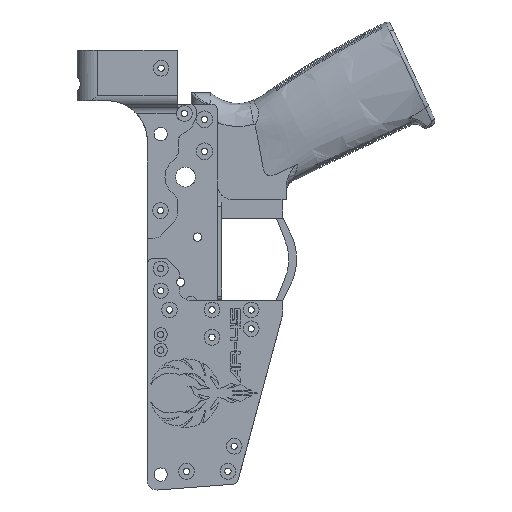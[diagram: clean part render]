
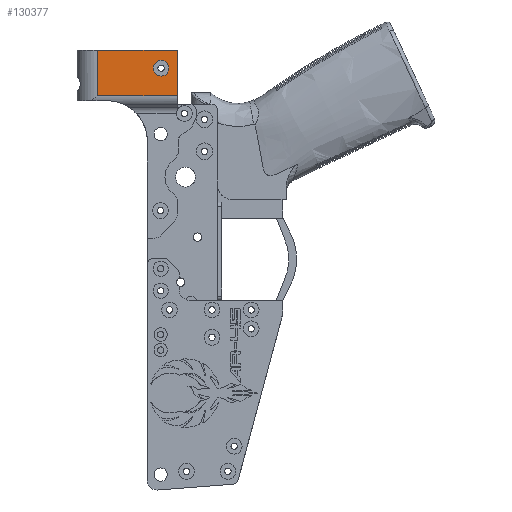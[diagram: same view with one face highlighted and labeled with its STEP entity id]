
A CAD part, left-side view. The second image highlights one B-rep face of the part: STEP entity #130377.
In plain terms, the highlighted planar face has unit normal (-1, 0, 0).
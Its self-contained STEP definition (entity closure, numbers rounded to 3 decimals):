
#2563 = CARTESIAN_POINT ( 'NONE',  ( -25., 7.678, -12.776 ) ) ;
#2951 = LINE ( 'NONE', #140693, #109962 ) ;
#7996 = EDGE_CURVE ( 'NONE', #59619, #16362, #136589, .T. ) ;
#9324 = AXIS2_PLACEMENT_3D ( 'NONE', #116725, #48260, #82517 ) ;
#12332 = EDGE_LOOP ( 'NONE', ( #117339, #46170 ) ) ;
#13072 = ORIENTED_EDGE ( 'NONE', *, *, #69360, .T. ) ;
#13967 = FACE_OUTER_BOUND ( 'NONE', #111401, .T. ) ;
#14723 = EDGE_CURVE ( 'NONE', #73125, #59619, #2951, .T. ) ;
#15175 = AXIS2_PLACEMENT_3D ( 'NONE', #59924, #96375, #49490 ) ;
#16362 = VERTEX_POINT ( 'NONE', #33906 ) ;
#18958 = CARTESIAN_POINT ( 'NONE',  ( -25., -30.202, -14.306 ) ) ;
#33906 = CARTESIAN_POINT ( 'NONE',  ( -25., 7.678, -10.291 ) ) ;
#35021 = CARTESIAN_POINT ( 'NONE',  ( -25., -22.502, 6.484 ) ) ;
#36368 = EDGE_CURVE ( 'NONE', #93127, #79195, #93649, .T. ) ;
#45684 = DIRECTION ( 'NONE',  ( -1., 0., 0. ) ) ;
#46170 = ORIENTED_EDGE ( 'NONE', *, *, #36368, .F. ) ;
#48260 = DIRECTION ( 'NONE',  ( 1., 0., 0. ) ) ;
#49490 = DIRECTION ( 'NONE',  ( 0., 0., 1. ) ) ;
#50831 = ORIENTED_EDGE ( 'NONE', *, *, #126546, .T. ) ;
#52582 = VECTOR ( 'NONE', #142627, 1000. ) ;
#58824 = VECTOR ( 'NONE', #123405, 1000. ) ;
#59619 = VERTEX_POINT ( 'NONE', #101866 ) ;
#59924 = CARTESIAN_POINT ( 'NONE',  ( -25., -22.502, 2.734 ) ) ;
#64695 = ORIENTED_EDGE ( 'NONE', *, *, #14723, .T. ) ;
#69360 = EDGE_CURVE ( 'NONE', #131514, #73125, #86780, .T. ) ;
#73125 = VERTEX_POINT ( 'NONE', #139478 ) ;
#76999 = DIRECTION ( 'NONE',  ( 0., 0., 1. ) ) ;
#79195 = VERTEX_POINT ( 'NONE', #35021 ) ;
#80540 = EDGE_CURVE ( 'NONE', #79195, #93127, #87482, .T. ) ;
#81036 = PLANE ( 'NONE',  #9324 ) ;
#82517 = DIRECTION ( 'NONE',  ( 0., 0., -1. ) ) ;
#86780 = LINE ( 'NONE', #18958, #52582 ) ;
#87482 = CIRCLE ( 'NONE', #111239, 3.75 ) ;
#90685 = CARTESIAN_POINT ( 'NONE',  ( -25., -36.779, -10.291 ) ) ;
#92203 = FACE_BOUND ( 'NONE', #12332, .T. ) ;
#93127 = VERTEX_POINT ( 'NONE', #114815 ) ;
#93431 = DIRECTION ( 'NONE',  ( 0., 0., -1. ) ) ;
#93649 = CIRCLE ( 'NONE', #15175, 3.75 ) ;
#96375 = DIRECTION ( 'NONE',  ( -1., 0., 0. ) ) ;
#101550 = ORIENTED_EDGE ( 'NONE', *, *, #7996, .T. ) ;
#101866 = CARTESIAN_POINT ( 'NONE',  ( -25., 7.678, 11.224 ) ) ;
#102276 = CARTESIAN_POINT ( 'NONE',  ( -25., -22.502, 2.734 ) ) ;
#107171 = DIRECTION ( 'NONE',  ( 0., 1., 0. ) ) ;
#109962 = VECTOR ( 'NONE', #107171, 1000. ) ;
#111239 = AXIS2_PLACEMENT_3D ( 'NONE', #102276, #45684, #76999 ) ;
#111401 = EDGE_LOOP ( 'NONE', ( #101550, #50831, #13072, #64695 ) ) ;
#111511 = LINE ( 'NONE', #90685, #58824 ) ;
#114815 = CARTESIAN_POINT ( 'NONE',  ( -25., -22.502, -1.016 ) ) ;
#115073 = VECTOR ( 'NONE', #93431, 1000. ) ;
#116725 = CARTESIAN_POINT ( 'NONE',  ( -25., -36.779, -288600.29 ) ) ;
#117339 = ORIENTED_EDGE ( 'NONE', *, *, #80540, .F. ) ;
#123405 = DIRECTION ( 'NONE',  ( 0., -1., 0. ) ) ;
#126546 = EDGE_CURVE ( 'NONE', #16362, #131514, #111511, .T. ) ;
#130377 = ADVANCED_FACE ( 'NONE', ( #92203, #13967 ), #81036, .F. ) ;
#131514 = VERTEX_POINT ( 'NONE', #144943 ) ;
#136589 = LINE ( 'NONE', #2563, #115073 ) ;
#139478 = CARTESIAN_POINT ( 'NONE',  ( -25., -30.202, 11.224 ) ) ;
#140693 = CARTESIAN_POINT ( 'NONE',  ( -25., -36.779, 11.224 ) ) ;
#142627 = DIRECTION ( 'NONE',  ( 0., 0., 1. ) ) ;
#144943 = CARTESIAN_POINT ( 'NONE',  ( -25., -30.202, -10.291 ) ) ;
